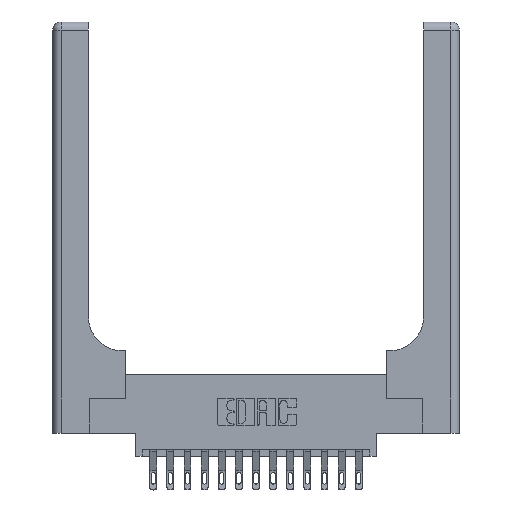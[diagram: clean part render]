
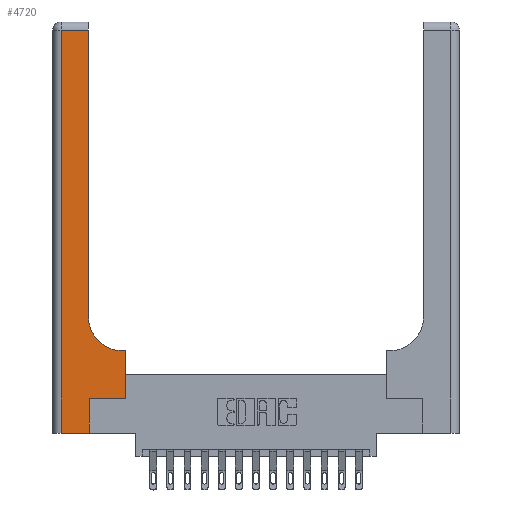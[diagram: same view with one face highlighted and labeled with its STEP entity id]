
A CAD part, top view. The second image highlights one B-rep face of the part: STEP entity #4720.
In plain terms, the highlighted planar face has unit normal (0, 0, 1).
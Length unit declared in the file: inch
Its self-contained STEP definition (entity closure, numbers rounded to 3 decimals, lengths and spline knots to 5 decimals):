
#242 = CARTESIAN_POINT ( 'NONE',  ( 0.265, 0.25, 0.37 ) ) ;
#311 = DIRECTION ( 'NONE',  ( 0., 1., 0. ) ) ;
#598 = CARTESIAN_POINT ( 'NONE',  ( 0., 0., 0.37 ) ) ;
#1027 = VECTOR ( 'NONE', #5030, 39.37008 ) ;
#1034 = FACE_OUTER_BOUND ( 'NONE', #6900, .T. ) ;
#1340 = EDGE_CURVE ( 'NONE', #9813, #3047, #17510, .T. ) ;
#1530 = VECTOR ( 'NONE', #311, 39.37008 ) ;
#1665 = DIRECTION ( 'NONE',  ( 1., 0., 0. ) ) ;
#1707 = DIRECTION ( 'NONE',  ( -1., 0., 0. ) ) ;
#1815 = EDGE_CURVE ( 'NONE', #17141, #3262, #13887, .T. ) ;
#1855 = ORIENTED_EDGE ( 'NONE', *, *, #17564, .T. ) ;
#2001 = CARTESIAN_POINT ( 'NONE',  ( 0.265, 0., 0.37 ) ) ;
#2249 = EDGE_CURVE ( 'NONE', #12963, #17380, #14719, .T. ) ;
#2515 = CARTESIAN_POINT ( 'NONE',  ( 0.265, 0., 0.37 ) ) ;
#2763 = CARTESIAN_POINT ( 'NONE',  ( 0.06, 3., 0.37 ) ) ;
#3001 = AXIS2_PLACEMENT_3D ( 'NONE', #3383, #13196, #4821 ) ;
#3044 = CIRCLE ( 'NONE', #3001, 0.25 ) ;
#3047 = VERTEX_POINT ( 'NONE', #4288 ) ;
#3101 = LINE ( 'NONE', #598, #6434 ) ;
#3249 = CARTESIAN_POINT ( 'NONE',  ( 0.26, 0.85, 0.37 ) ) ;
#3262 = VERTEX_POINT ( 'NONE', #15959 ) ;
#3345 = ORIENTED_EDGE ( 'NONE', *, *, #9856, .T. ) ;
#3383 = CARTESIAN_POINT ( 'NONE',  ( 0.51, 0.85, 0.37 ) ) ;
#4288 = CARTESIAN_POINT ( 'NONE',  ( 0.528, 0.25, 0.37 ) ) ;
#4320 = CARTESIAN_POINT ( 'NONE',  ( 0.26, 2.94, 0.37 ) ) ;
#4720 = ADVANCED_FACE ( 'NONE', ( #1034 ), #13709, .F. ) ;
#4821 = DIRECTION ( 'NONE',  ( 1., 0., 0. ) ) ;
#4851 = DIRECTION ( 'NONE',  ( 1., 0., 0. ) ) ;
#5030 = DIRECTION ( 'NONE',  ( -1., 0., 0. ) ) ;
#5288 = CARTESIAN_POINT ( 'NONE',  ( 0., 3., 0.37 ) ) ;
#5315 = ORIENTED_EDGE ( 'NONE', *, *, #1815, .T. ) ;
#6434 = VECTOR ( 'NONE', #4851, 39.37008 ) ;
#6789 = DIRECTION ( 'NONE',  ( -1., 0., 0. ) ) ;
#6791 = CARTESIAN_POINT ( 'NONE',  ( 0.528, 0.6, 0.37 ) ) ;
#6840 = ORIENTED_EDGE ( 'NONE', *, *, #15963, .T. ) ;
#6900 = EDGE_LOOP ( 'NONE', ( #11279, #3345, #5315, #10044, #8018, #16398, #6840, #14798, #1855 ) ) ;
#7078 = DIRECTION ( 'NONE',  ( 0., -1., 0. ) ) ;
#7688 = VERTEX_POINT ( 'NONE', #12082 ) ;
#7829 = VECTOR ( 'NONE', #17742, 39.37008 ) ;
#8018 = ORIENTED_EDGE ( 'NONE', *, *, #8521, .T. ) ;
#8168 = CARTESIAN_POINT ( 'NONE',  ( 0.26, 3., 0.37 ) ) ;
#8521 = EDGE_CURVE ( 'NONE', #17604, #9813, #17021, .T. ) ;
#8809 = CARTESIAN_POINT ( 'NONE',  ( 0.26, 0.6, 0.37 ) ) ;
#9203 = CARTESIAN_POINT ( 'NONE',  ( 0., 2.94, 0.37 ) ) ;
#9384 = VECTOR ( 'NONE', #1665, 39.37008 ) ;
#9813 = VERTEX_POINT ( 'NONE', #13349 ) ;
#9856 = EDGE_CURVE ( 'NONE', #17380, #17141, #15914, .T. ) ;
#10044 = ORIENTED_EDGE ( 'NONE', *, *, #16129, .T. ) ;
#10950 = DIRECTION ( 'NONE',  ( 0., 1., 0. ) ) ;
#11279 = ORIENTED_EDGE ( 'NONE', *, *, #2249, .T. ) ;
#12082 = CARTESIAN_POINT ( 'NONE',  ( 0.51, 0.6, 0.37 ) ) ;
#12291 = LINE ( 'NONE', #8809, #15918 ) ;
#12963 = VERTEX_POINT ( 'NONE', #3249 ) ;
#13196 = DIRECTION ( 'NONE',  ( 0., 0., -1. ) ) ;
#13349 = CARTESIAN_POINT ( 'NONE',  ( 0.265, 0.25, 0.37 ) ) ;
#13403 = VECTOR ( 'NONE', #10950, 39.37008 ) ;
#13709 = PLANE ( 'NONE',  #17436 ) ;
#13887 = LINE ( 'NONE', #2763, #17496 ) ;
#14719 = LINE ( 'NONE', #8168, #7829 ) ;
#14798 = ORIENTED_EDGE ( 'NONE', *, *, #17418, .T. ) ;
#15075 = DIRECTION ( 'NONE',  ( 0., 0., -1. ) ) ;
#15683 = VERTEX_POINT ( 'NONE', #6791 ) ;
#15914 = LINE ( 'NONE', #9203, #1027 ) ;
#15918 = VECTOR ( 'NONE', #1707, 39.37008 ) ;
#15959 = CARTESIAN_POINT ( 'NONE',  ( 0.06, 0., 0.37 ) ) ;
#15963 = EDGE_CURVE ( 'NONE', #3047, #15683, #15967, .T. ) ;
#15967 = LINE ( 'NONE', #17035, #1530 ) ;
#16129 = EDGE_CURVE ( 'NONE', #3262, #17604, #3101, .T. ) ;
#16236 = CARTESIAN_POINT ( 'NONE',  ( 0.06, 2.94, 0.37 ) ) ;
#16398 = ORIENTED_EDGE ( 'NONE', *, *, #1340, .T. ) ;
#17021 = LINE ( 'NONE', #2515, #13403 ) ;
#17035 = CARTESIAN_POINT ( 'NONE',  ( 0.528, 0.25, 0.37 ) ) ;
#17141 = VERTEX_POINT ( 'NONE', #16236 ) ;
#17380 = VERTEX_POINT ( 'NONE', #4320 ) ;
#17418 = EDGE_CURVE ( 'NONE', #15683, #7688, #12291, .T. ) ;
#17436 = AXIS2_PLACEMENT_3D ( 'NONE', #5288, #15075, #6789 ) ;
#17496 = VECTOR ( 'NONE', #7078, 39.37008 ) ;
#17510 = LINE ( 'NONE', #242, #9384 ) ;
#17564 = EDGE_CURVE ( 'NONE', #7688, #12963, #3044, .T. ) ;
#17604 = VERTEX_POINT ( 'NONE', #2001 ) ;
#17742 = DIRECTION ( 'NONE',  ( 0., 1., 0. ) ) ;
